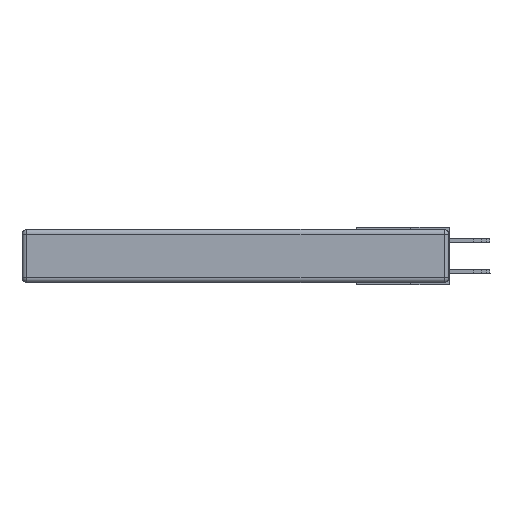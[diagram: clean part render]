
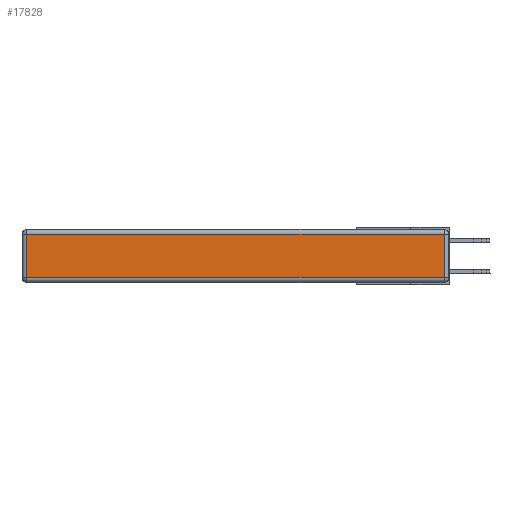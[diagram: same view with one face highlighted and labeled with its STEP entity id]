
A CAD part, left-side view. The second image highlights one B-rep face of the part: STEP entity #17828.
In plain terms, the highlighted planar face has unit normal (-1, 0, 0).
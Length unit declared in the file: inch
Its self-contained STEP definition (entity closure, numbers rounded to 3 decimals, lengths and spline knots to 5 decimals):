
#299 = CARTESIAN_POINT ( 'NONE',  ( 0., 0.03, -0.313 ) ) ;
#1651 = AXIS2_PLACEMENT_3D ( 'NONE', #4709, #18735, #9926 ) ;
#1656 = VECTOR ( 'NONE', #8877, 39.37008 ) ;
#2101 = ORIENTED_EDGE ( 'NONE', *, *, #13396, .T. ) ;
#2350 = DIRECTION ( 'NONE',  ( 0., 1., 0. ) ) ;
#3678 = EDGE_CURVE ( 'NONE', #17527, #4561, #17460, .T. ) ;
#4208 = FACE_OUTER_BOUND ( 'NONE', #8941, .T. ) ;
#4431 = VECTOR ( 'NONE', #2350, 39.37008 ) ;
#4561 = VERTEX_POINT ( 'NONE', #20298 ) ;
#4709 = CARTESIAN_POINT ( 'NONE',  ( 0., 0., -0.343 ) ) ;
#4718 = ORIENTED_EDGE ( 'NONE', *, *, #3678, .T. ) ;
#5283 = CARTESIAN_POINT ( 'NONE',  ( 0., 2.72, -0.343 ) ) ;
#5328 = VECTOR ( 'NONE', #21094, 39.37008 ) ;
#8032 = CARTESIAN_POINT ( 'NONE',  ( 0., 0.03, -0.343 ) ) ;
#8877 = DIRECTION ( 'NONE',  ( 0., 0., -1. ) ) ;
#8941 = EDGE_LOOP ( 'NONE', ( #20172, #4718, #2101, #20653 ) ) ;
#9926 = DIRECTION ( 'NONE',  ( 0., 0., 1. ) ) ;
#9979 = VERTEX_POINT ( 'NONE', #17342 ) ;
#11416 = LINE ( 'NONE', #20104, #4431 ) ;
#13395 = VERTEX_POINT ( 'NONE', #15093 ) ;
#13396 = EDGE_CURVE ( 'NONE', #4561, #13395, #11416, .T. ) ;
#13433 = LINE ( 'NONE', #17516, #5328 ) ;
#14060 = EDGE_CURVE ( 'NONE', #13395, #9979, #15818, .T. ) ;
#15093 = CARTESIAN_POINT ( 'NONE',  ( 0., 2.72, -0.03 ) ) ;
#15818 = LINE ( 'NONE', #5283, #1656 ) ;
#17203 = EDGE_CURVE ( 'NONE', #9979, #17527, #13433, .T. ) ;
#17342 = CARTESIAN_POINT ( 'NONE',  ( 0., 2.72, -0.313 ) ) ;
#17460 = LINE ( 'NONE', #8032, #18987 ) ;
#17516 = CARTESIAN_POINT ( 'NONE',  ( 0., 0., -0.313 ) ) ;
#17527 = VERTEX_POINT ( 'NONE', #299 ) ;
#17828 = ADVANCED_FACE ( 'NONE', ( #4208 ), #20614, .T. ) ;
#18735 = DIRECTION ( 'NONE',  ( -1., 0., 0. ) ) ;
#18987 = VECTOR ( 'NONE', #20448, 39.37008 ) ;
#20104 = CARTESIAN_POINT ( 'NONE',  ( 0., 2.75, -0.03 ) ) ;
#20172 = ORIENTED_EDGE ( 'NONE', *, *, #17203, .T. ) ;
#20298 = CARTESIAN_POINT ( 'NONE',  ( 0., 0.03, -0.03 ) ) ;
#20448 = DIRECTION ( 'NONE',  ( 0., 0., 1. ) ) ;
#20614 = PLANE ( 'NONE',  #1651 ) ;
#20653 = ORIENTED_EDGE ( 'NONE', *, *, #14060, .T. ) ;
#21094 = DIRECTION ( 'NONE',  ( 0., -1., 0. ) ) ;
